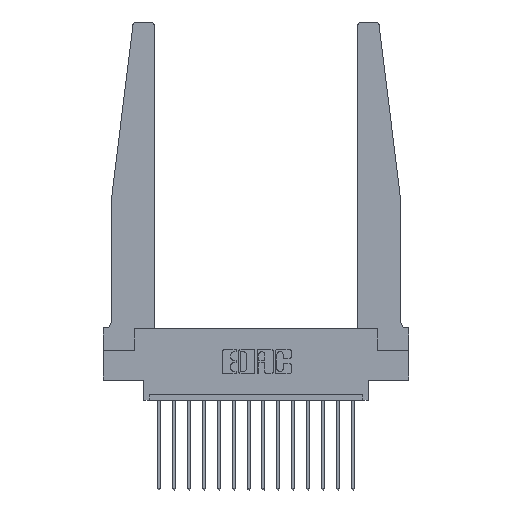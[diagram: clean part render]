
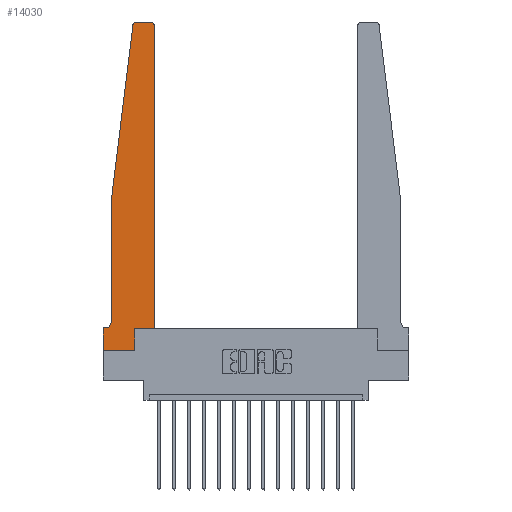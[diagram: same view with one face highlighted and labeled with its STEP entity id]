
A CAD part, top view. The second image highlights one B-rep face of the part: STEP entity #14030.
In plain terms, the highlighted planar face has unit normal (0, 0, 1).
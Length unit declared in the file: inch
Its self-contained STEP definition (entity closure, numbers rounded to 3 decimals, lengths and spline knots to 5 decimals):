
#63 = DIRECTION ( 'NONE',  ( 1., 0., 0. ) ) ;
#205 = CARTESIAN_POINT ( 'NONE',  ( 0.395, 2.75, 0.37 ) ) ;
#216 = LINE ( 'NONE', #12873, #3595 ) ;
#311 = LINE ( 'NONE', #1893, #13950 ) ;
#508 = LINE ( 'NONE', #3427, #949 ) ;
#949 = VECTOR ( 'NONE', #1211, 39.37008 ) ;
#1211 = DIRECTION ( 'NONE',  ( 0., -1., 0. ) ) ;
#1453 = EDGE_CURVE ( 'NONE', #13609, #15819, #311, .T. ) ;
#1593 = VERTEX_POINT ( 'NONE', #13673 ) ;
#1657 = EDGE_CURVE ( 'NONE', #1593, #4156, #508, .T. ) ;
#1781 = CIRCLE ( 'NONE', #7036, 0.03 ) ;
#1893 = CARTESIAN_POINT ( 'NONE',  ( 0.2605, 0.18, 0.37 ) ) ;
#2071 = DIRECTION ( 'NONE',  ( 1., 0., 0. ) ) ;
#2187 = DIRECTION ( 'NONE',  ( 0., 0., 1. ) ) ;
#2213 = ORIENTED_EDGE ( 'NONE', *, *, #14923, .T. ) ;
#2527 = DIRECTION ( 'NONE',  ( -1., 0., 0. ) ) ;
#2885 = VERTEX_POINT ( 'NONE', #13048 ) ;
#3064 = PLANE ( 'NONE',  #8434 ) ;
#3111 = EDGE_CURVE ( 'NONE', #2885, #16439, #10790, .T. ) ;
#3427 = CARTESIAN_POINT ( 'NONE',  ( 0.065, 1.25, 0.37 ) ) ;
#3433 = EDGE_CURVE ( 'NONE', #5364, #8582, #4095, .T. ) ;
#3595 = VECTOR ( 'NONE', #8841, 39.37008 ) ;
#3985 = CARTESIAN_POINT ( 'NONE',  ( 0.27653, 2.75, 0.37 ) ) ;
#4095 = CIRCLE ( 'NONE', #9020, 0.03 ) ;
#4156 = VERTEX_POINT ( 'NONE', #14869 ) ;
#4254 = CARTESIAN_POINT ( 'NONE',  ( 0., 0.1875, 0.37 ) ) ;
#4685 = DIRECTION ( 'NONE',  ( 1., 0., 0. ) ) ;
#4724 = ORIENTED_EDGE ( 'NONE', *, *, #5757, .T. ) ;
#5364 = VERTEX_POINT ( 'NONE', #3985 ) ;
#5515 = CARTESIAN_POINT ( 'NONE',  ( 0.425, 0.18, 0.37 ) ) ;
#5623 = ORIENTED_EDGE ( 'NONE', *, *, #17037, .T. ) ;
#5757 = EDGE_CURVE ( 'NONE', #15819, #11266, #9214, .T. ) ;
#5820 = CARTESIAN_POINT ( 'NONE',  ( 0., 0.1875, 0.37 ) ) ;
#6249 = VERTEX_POINT ( 'NONE', #205 ) ;
#6288 = CARTESIAN_POINT ( 'NONE',  ( 0.395, 2.72, 0.37 ) ) ;
#6343 = EDGE_CURVE ( 'NONE', #8582, #1593, #9615, .T. ) ;
#6454 = ORIENTED_EDGE ( 'NONE', *, *, #10903, .T. ) ;
#6476 = DIRECTION ( 'NONE',  ( -1., 0., 0. ) ) ;
#6749 = CARTESIAN_POINT ( 'NONE',  ( 0., 0., 0.37 ) ) ;
#7036 = AXIS2_PLACEMENT_3D ( 'NONE', #6288, #2187, #8982 ) ;
#7333 = VECTOR ( 'NONE', #16714, 39.37008 ) ;
#7382 = LINE ( 'NONE', #6749, #17267 ) ;
#7661 = ORIENTED_EDGE ( 'NONE', *, *, #8742, .T. ) ;
#7745 = FACE_OUTER_BOUND ( 'NONE', #11941, .T. ) ;
#8357 = LINE ( 'NONE', #12561, #7333 ) ;
#8434 = AXIS2_PLACEMENT_3D ( 'NONE', #5820, #12819, #4685 ) ;
#8582 = VERTEX_POINT ( 'NONE', #17055 ) ;
#8668 = VECTOR ( 'NONE', #6476, 39.37008 ) ;
#8742 = EDGE_CURVE ( 'NONE', #9844, #6249, #1781, .T. ) ;
#8841 = DIRECTION ( 'NONE',  ( 0., 1., 0. ) ) ;
#8923 = CARTESIAN_POINT ( 'NONE',  ( 0.065, 1.25, 0.37 ) ) ;
#8982 = DIRECTION ( 'NONE',  ( 1., 0., 0. ) ) ;
#9020 = AXIS2_PLACEMENT_3D ( 'NONE', #13802, #13855, #2071 ) ;
#9121 = EDGE_CURVE ( 'NONE', #11308, #13609, #11001, .T. ) ;
#9207 = DIRECTION ( 'NONE',  ( 0., 0., -1. ) ) ;
#9214 = LINE ( 'NONE', #5515, #16143 ) ;
#9615 = LINE ( 'NONE', #8923, #17184 ) ;
#9844 = VERTEX_POINT ( 'NONE', #14251 ) ;
#10427 = ORIENTED_EDGE ( 'NONE', *, *, #1657, .T. ) ;
#10790 = LINE ( 'NONE', #13069, #8668 ) ;
#10903 = EDGE_CURVE ( 'NONE', #16439, #11308, #7382, .T. ) ;
#10994 = CARTESIAN_POINT ( 'NONE',  ( 0.425, 0.18, 0.37 ) ) ;
#11001 = LINE ( 'NONE', #13341, #12878 ) ;
#11257 = DIRECTION ( 'NONE',  ( 0., 1., 0. ) ) ;
#11266 = VERTEX_POINT ( 'NONE', #10994 ) ;
#11308 = VERTEX_POINT ( 'NONE', #16756 ) ;
#11492 = ORIENTED_EDGE ( 'NONE', *, *, #12046, .T. ) ;
#11598 = DIRECTION ( 'NONE',  ( -0.122, -0.992, 0. ) ) ;
#11941 = EDGE_LOOP ( 'NONE', ( #11492, #13603, #13377, #10427, #5623, #15596, #6454, #16989, #15578, #4724, #2213, #7661 ) ) ;
#11972 = AXIS2_PLACEMENT_3D ( 'NONE', #15894, #9207, #2527 ) ;
#12046 = EDGE_CURVE ( 'NONE', #6249, #5364, #8357, .T. ) ;
#12420 = CARTESIAN_POINT ( 'NONE',  ( 0.2605, 0.18, 0.37 ) ) ;
#12561 = CARTESIAN_POINT ( 'NONE',  ( 0.25, 2.75, 0.37 ) ) ;
#12819 = DIRECTION ( 'NONE',  ( 0., 0., 1. ) ) ;
#12873 = CARTESIAN_POINT ( 'NONE',  ( 0.425, 0.18, 0.37 ) ) ;
#12878 = VECTOR ( 'NONE', #17368, 39.37008 ) ;
#13048 = CARTESIAN_POINT ( 'NONE',  ( 0.015, 0.1875, 0.37 ) ) ;
#13069 = CARTESIAN_POINT ( 'NONE',  ( 0.065, 0.1875, 0.37 ) ) ;
#13341 = CARTESIAN_POINT ( 'NONE',  ( 0., 0., 0.37 ) ) ;
#13377 = ORIENTED_EDGE ( 'NONE', *, *, #6343, .T. ) ;
#13603 = ORIENTED_EDGE ( 'NONE', *, *, #3433, .T. ) ;
#13609 = VERTEX_POINT ( 'NONE', #15626 ) ;
#13673 = CARTESIAN_POINT ( 'NONE',  ( 0.065, 1.25, 0.37 ) ) ;
#13802 = CARTESIAN_POINT ( 'NONE',  ( 0.27653, 2.72, 0.37 ) ) ;
#13855 = DIRECTION ( 'NONE',  ( 0., 0., 1. ) ) ;
#13950 = VECTOR ( 'NONE', #11257, 39.37008 ) ;
#14030 = ADVANCED_FACE ( 'NONE', ( #7745 ), #3064, .T. ) ;
#14251 = CARTESIAN_POINT ( 'NONE',  ( 0.425, 2.72, 0.37 ) ) ;
#14869 = CARTESIAN_POINT ( 'NONE',  ( 0.065, 0.2375, 0.37 ) ) ;
#14923 = EDGE_CURVE ( 'NONE', #11266, #9844, #216, .T. ) ;
#15495 = DIRECTION ( 'NONE',  ( 0., -1., 0. ) ) ;
#15578 = ORIENTED_EDGE ( 'NONE', *, *, #1453, .T. ) ;
#15596 = ORIENTED_EDGE ( 'NONE', *, *, #3111, .T. ) ;
#15626 = CARTESIAN_POINT ( 'NONE',  ( 0.2605, 0., 0.37 ) ) ;
#15819 = VERTEX_POINT ( 'NONE', #12420 ) ;
#15894 = CARTESIAN_POINT ( 'NONE',  ( 0.015, 0.2375, 0.37 ) ) ;
#16143 = VECTOR ( 'NONE', #63, 39.37008 ) ;
#16439 = VERTEX_POINT ( 'NONE', #4254 ) ;
#16502 = CIRCLE ( 'NONE', #11972, 0.05 ) ;
#16714 = DIRECTION ( 'NONE',  ( -1., 0., 0. ) ) ;
#16756 = CARTESIAN_POINT ( 'NONE',  ( 0., 0., 0.37 ) ) ;
#16989 = ORIENTED_EDGE ( 'NONE', *, *, #9121, .T. ) ;
#17037 = EDGE_CURVE ( 'NONE', #4156, #2885, #16502, .T. ) ;
#17055 = CARTESIAN_POINT ( 'NONE',  ( 0.24675, 2.72367, 0.37 ) ) ;
#17184 = VECTOR ( 'NONE', #11598, 39.37008 ) ;
#17267 = VECTOR ( 'NONE', #15495, 39.37008 ) ;
#17368 = DIRECTION ( 'NONE',  ( 1., 0., 0. ) ) ;
